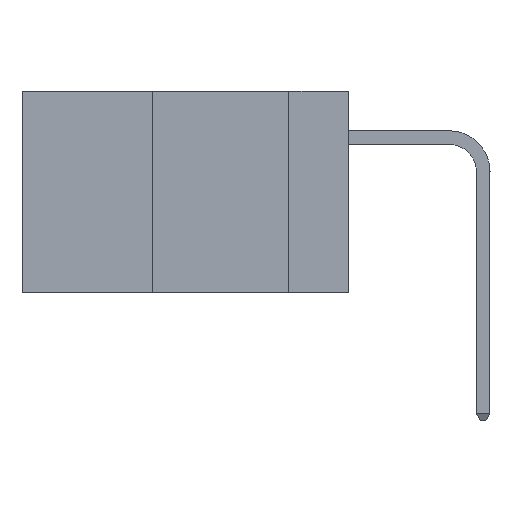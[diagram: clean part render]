
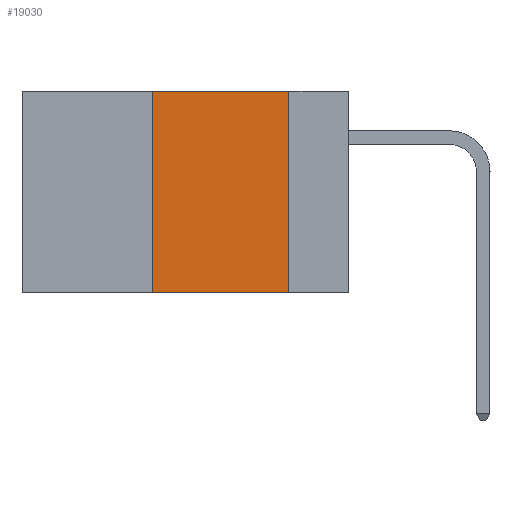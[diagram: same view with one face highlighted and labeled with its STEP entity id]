
A CAD part, left-side view. The second image highlights one B-rep face of the part: STEP entity #19030.
In plain terms, the highlighted planar face has unit normal (-1, 0, 0).
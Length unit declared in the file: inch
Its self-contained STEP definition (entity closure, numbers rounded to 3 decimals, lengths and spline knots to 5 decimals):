
#1646 = CARTESIAN_POINT ( 'NONE',  ( 0., 0.36, -0.37 ) ) ;
#1796 = EDGE_CURVE ( 'NONE', #12821, #28465, #21168, .T. ) ;
#2297 = DIRECTION ( 'NONE',  ( 0., 0., -1. ) ) ;
#2543 = CARTESIAN_POINT ( 'NONE',  ( 0., 0.11, 0. ) ) ;
#2903 = LINE ( 'NONE', #25751, #9764 ) ;
#3070 = EDGE_LOOP ( 'NONE', ( #36901, #22722, #20522, #7699 ) ) ;
#5580 = VECTOR ( 'NONE', #34630, 39.37008 ) ;
#5930 = CARTESIAN_POINT ( 'NONE',  ( 0., 0.36, 0. ) ) ;
#6728 = FACE_OUTER_BOUND ( 'NONE', #3070, .T. ) ;
#7699 = ORIENTED_EDGE ( 'NONE', *, *, #1796, .T. ) ;
#9013 = CARTESIAN_POINT ( 'NONE',  ( 0., 0.11, 0. ) ) ;
#9406 = EDGE_CURVE ( 'NONE', #19083, #28465, #10256, .T. ) ;
#9764 = VECTOR ( 'NONE', #31638, 39.37008 ) ;
#10256 = LINE ( 'NONE', #9013, #17132 ) ;
#12821 = VERTEX_POINT ( 'NONE', #1646 ) ;
#13951 = PLANE ( 'NONE',  #18968 ) ;
#16887 = CARTESIAN_POINT ( 'NONE',  ( 0., 0.6, 0. ) ) ;
#17132 = VECTOR ( 'NONE', #35398, 39.37008 ) ;
#18342 = VERTEX_POINT ( 'NONE', #5930 ) ;
#18968 = AXIS2_PLACEMENT_3D ( 'NONE', #16887, #19843, #2297 ) ;
#18993 = EDGE_CURVE ( 'NONE', #18342, #19083, #30106, .T. ) ;
#19030 = ADVANCED_FACE ( 'NONE', ( #6728 ), #13951, .F. ) ;
#19083 = VERTEX_POINT ( 'NONE', #2543 ) ;
#19843 = DIRECTION ( 'NONE',  ( 1., 0., 0. ) ) ;
#20043 = CARTESIAN_POINT ( 'NONE',  ( 0., 0.6, -0.37 ) ) ;
#20522 = ORIENTED_EDGE ( 'NONE', *, *, #22451, .F. ) ;
#21168 = LINE ( 'NONE', #20043, #5580 ) ;
#22451 = EDGE_CURVE ( 'NONE', #12821, #18342, #2903, .T. ) ;
#22722 = ORIENTED_EDGE ( 'NONE', *, *, #18993, .F. ) ;
#25751 = CARTESIAN_POINT ( 'NONE',  ( 0., 0.36, 0. ) ) ;
#28465 = VERTEX_POINT ( 'NONE', #36107 ) ;
#30106 = LINE ( 'NONE', #31344, #37007 ) ;
#31344 = CARTESIAN_POINT ( 'NONE',  ( 0., 0.6, 0. ) ) ;
#31638 = DIRECTION ( 'NONE',  ( 0., 0., 1. ) ) ;
#34295 = DIRECTION ( 'NONE',  ( 0., -1., 0. ) ) ;
#34630 = DIRECTION ( 'NONE',  ( 0., -1., 0. ) ) ;
#35398 = DIRECTION ( 'NONE',  ( 0., 0., -1. ) ) ;
#36107 = CARTESIAN_POINT ( 'NONE',  ( 0., 0.11, -0.37 ) ) ;
#36901 = ORIENTED_EDGE ( 'NONE', *, *, #9406, .F. ) ;
#37007 = VECTOR ( 'NONE', #34295, 39.37008 ) ;
